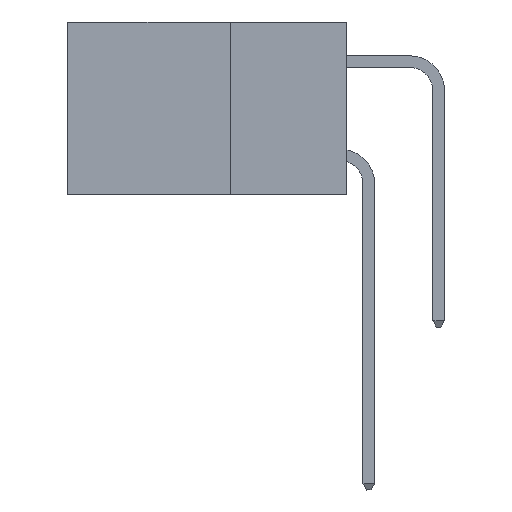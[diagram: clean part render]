
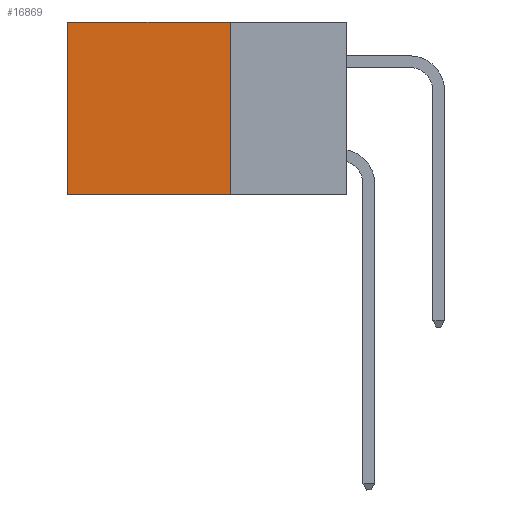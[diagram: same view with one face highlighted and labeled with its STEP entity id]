
A CAD part, left-side view. The second image highlights one B-rep face of the part: STEP entity #16869.
In plain terms, the highlighted planar face has unit normal (-1, 0, 0).
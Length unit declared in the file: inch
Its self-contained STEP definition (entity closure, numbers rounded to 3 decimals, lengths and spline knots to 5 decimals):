
#2149 = LINE ( 'NONE', #31905, #8003 ) ;
#4187 = VECTOR ( 'NONE', #18313, 39.37008 ) ;
#6154 = AXIS2_PLACEMENT_3D ( 'NONE', #28147, #28274, #10574 ) ;
#6753 = ORIENTED_EDGE ( 'NONE', *, *, #29171, .T. ) ;
#7730 = VERTEX_POINT ( 'NONE', #15932 ) ;
#8003 = VECTOR ( 'NONE', #12210, 39.37008 ) ;
#8885 = ORIENTED_EDGE ( 'NONE', *, *, #21367, .F. ) ;
#9668 = EDGE_CURVE ( 'NONE', #29470, #14855, #15895, .T. ) ;
#10574 = DIRECTION ( 'NONE',  ( 0., 0., -1. ) ) ;
#10748 = LINE ( 'NONE', #32744, #32655 ) ;
#12210 = DIRECTION ( 'NONE',  ( 0., 0., -1. ) ) ;
#13854 = VERTEX_POINT ( 'NONE', #24864 ) ;
#14855 = VERTEX_POINT ( 'NONE', #30893 ) ;
#15075 = FACE_OUTER_BOUND ( 'NONE', #26721, .T. ) ;
#15895 = LINE ( 'NONE', #20296, #35577 ) ;
#15932 = CARTESIAN_POINT ( 'NONE',  ( 0.2875, 0.25, 0. ) ) ;
#16869 = ADVANCED_FACE ( 'NONE', ( #15075 ), #25248, .F. ) ;
#18313 = DIRECTION ( 'NONE',  ( 0., 0., -1. ) ) ;
#18531 = DIRECTION ( 'NONE',  ( 0., 1., 0. ) ) ;
#18941 = CARTESIAN_POINT ( 'NONE',  ( 0.2875, 0.25, -0.37 ) ) ;
#20296 = CARTESIAN_POINT ( 'NONE',  ( 0.2875, 0.25, -0.37 ) ) ;
#20418 = LINE ( 'NONE', #24345, #4187 ) ;
#21367 = EDGE_CURVE ( 'NONE', #7730, #29470, #2149, .T. ) ;
#22485 = ORIENTED_EDGE ( 'NONE', *, *, #26441, .T. ) ;
#24345 = CARTESIAN_POINT ( 'NONE',  ( 0.2875, 0.6, 0. ) ) ;
#24864 = CARTESIAN_POINT ( 'NONE',  ( 0.2875, 0.6, 0. ) ) ;
#25248 = PLANE ( 'NONE',  #6154 ) ;
#26441 = EDGE_CURVE ( 'NONE', #13854, #14855, #20418, .T. ) ;
#26721 = EDGE_LOOP ( 'NONE', ( #22485, #36309, #8885, #6753 ) ) ;
#28147 = CARTESIAN_POINT ( 'NONE',  ( 0.2875, 0.25, 0. ) ) ;
#28274 = DIRECTION ( 'NONE',  ( 1., 0., 0. ) ) ;
#29171 = EDGE_CURVE ( 'NONE', #7730, #13854, #10748, .T. ) ;
#29470 = VERTEX_POINT ( 'NONE', #18941 ) ;
#30893 = CARTESIAN_POINT ( 'NONE',  ( 0.2875, 0.6, -0.37 ) ) ;
#31503 = DIRECTION ( 'NONE',  ( 0., 1., 0. ) ) ;
#31905 = CARTESIAN_POINT ( 'NONE',  ( 0.2875, 0.25, 0. ) ) ;
#32655 = VECTOR ( 'NONE', #18531, 39.37008 ) ;
#32744 = CARTESIAN_POINT ( 'NONE',  ( 0.2875, 0.25, 0. ) ) ;
#35577 = VECTOR ( 'NONE', #31503, 39.37008 ) ;
#36309 = ORIENTED_EDGE ( 'NONE', *, *, #9668, .F. ) ;
